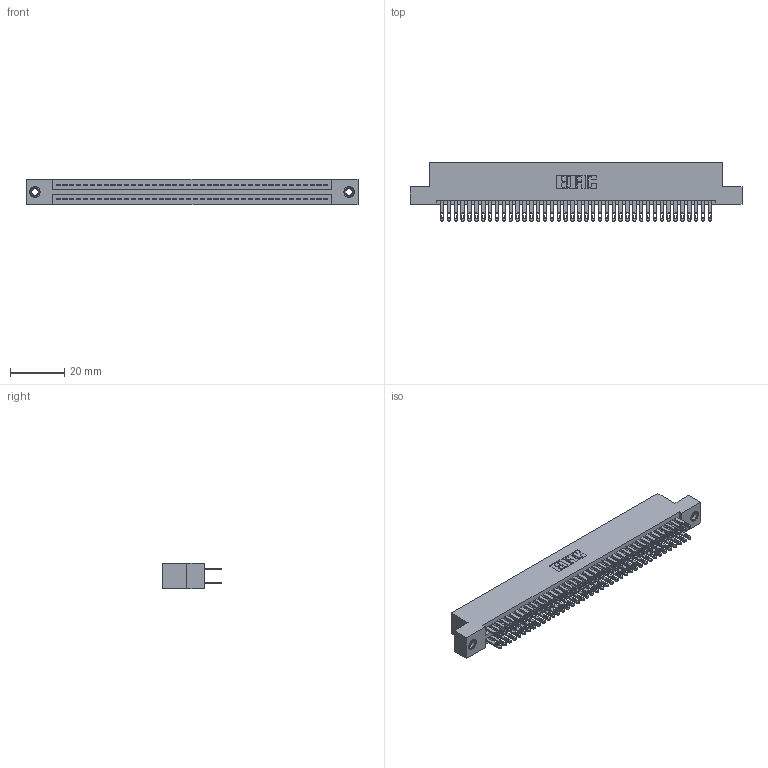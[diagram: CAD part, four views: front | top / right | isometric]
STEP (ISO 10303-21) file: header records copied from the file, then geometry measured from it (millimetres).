
FILE_DESCRIPTION (( 'STEP AP203' ), '1' );
FILE_NAME ('345-080-500-207.STEP', '2019-10-31T17:41:34', ( '' ), ( '' ), 'SwSTEP 2.0', 'SolidWorks 2016', '' );
FILE_SCHEMA (( 'CONFIG_CONTROL_DESIGN' ));
Length unit declared in the file: inch
Products named in the file (4): 345-250-001_345-250-005-103; 345-292-001_345-293-100; 345-080-500-207; 345 Part_Flush Mounting Lugs - 0.156 Dia-TI
Assembly tree (83 placements, depth 2):
  345-080-500-207
    345 Part_Flush Mounting Lugs - 0.156 Dia-TI
    345-292-001_345-293-100  x80
    345-250-001_345-250-005-103  x2
Bounding box: 122.81 x 21.51 x 9.4 mm (x, y, z)
Volume: 12142.2 mm3; surface area: 18753.3 mm2
Topology: 83 solids, 83 shells, 3866 faces, 11757 edges, 7830 vertices
Faces by surface type: plane 2272, cylinder 1578, cone 12, torus 4
Entity records: 32770 total; most frequent: CARTESIAN_POINT 5475, ORIENTED_EDGE 5402, DIRECTION 4859, EDGE_CURVE 2701, VECTOR 2385, LINE 2385, VERTEX_POINT 1796, AXIS2_PLACEMENT_3D 1237
